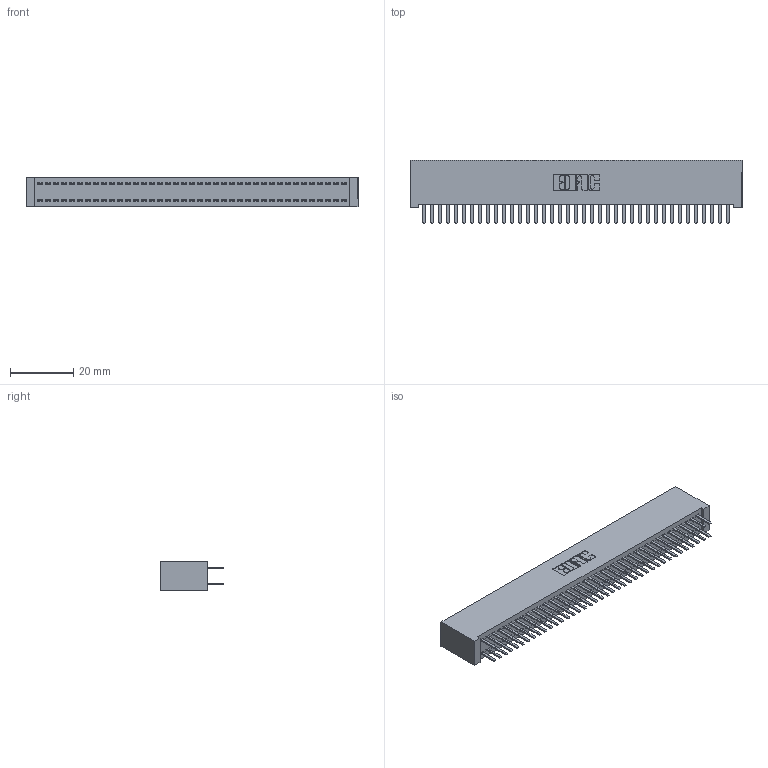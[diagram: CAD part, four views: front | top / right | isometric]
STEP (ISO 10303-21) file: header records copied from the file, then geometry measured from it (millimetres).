
FILE_DESCRIPTION (( 'STEP AP203' ), '1' );
FILE_NAME ('342-078-520-201.STEP', '2019-10-04T11:01:21', ( '' ), ( '' ), 'SwSTEP 2.0', 'SolidWorks 2016', '' );
FILE_SCHEMA (( 'CONFIG_CONTROL_DESIGN' ));
Length unit declared in the file: inch
Products named in the file (3): 345-292-001_345-293-120; 342-078-520-201; 342 Part_Lugless
Assembly tree (79 placements, depth 2):
  342-078-520-201
    342 Part_Lugless
    345-292-001_345-293-120  x78
Bounding box: 105.31 x 20.02 x 9.4 mm (x, y, z)
Volume: 9853 mm3; surface area: 16329.6 mm2
Topology: 79 solids, 79 shells, 4470 faces, 12989 edges, 8450 vertices
Faces by surface type: plane 3026, cylinder 1444
Entity records: 25183 total; most frequent: CARTESIAN_POINT 4186, ORIENTED_EDGE 4110, DIRECTION 3563, EDGE_CURVE 2055, LINE 1931, VECTOR 1931, VERTEX_POINT 1366, AXIS2_PLACEMENT_3D 816
